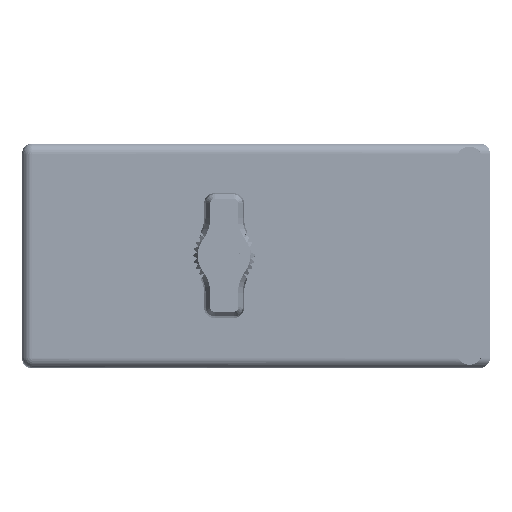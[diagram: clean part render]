
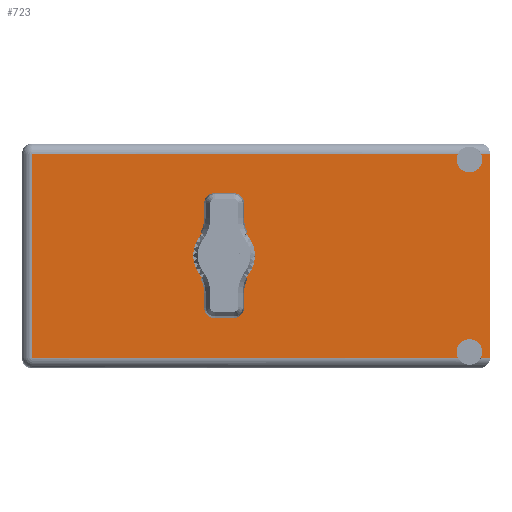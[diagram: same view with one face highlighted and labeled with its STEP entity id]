
A CAD part, top view. The second image highlights one B-rep face of the part: STEP entity #723.
In plain terms, the highlighted face is planar.
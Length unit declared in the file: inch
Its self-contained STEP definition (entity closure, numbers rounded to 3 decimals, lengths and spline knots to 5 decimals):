
#493 = LINE ( 'NONE', #103221, #78353 ) ;
#723 = ADVANCED_FACE ( 'NONE', ( #60271, #27135 ), #27679, .T. ) ;
#1004 = LINE ( 'NONE', #15747, #63517 ) ;
#2208 = EDGE_CURVE ( 'NONE', #18664, #69433, #89335, .T. ) ;
#5117 = EDGE_LOOP ( 'NONE', ( #17253, #62766 ) ) ;
#6814 = CARTESIAN_POINT ( 'NONE',  ( 1.75083, 1.93, -0.695 ) ) ;
#7413 = EDGE_CURVE ( 'NONE', #67430, #36402, #26645, .T. ) ;
#8121 = AXIS2_PLACEMENT_3D ( 'NONE', #72641, #79460, #87687 ) ;
#8572 = EDGE_CURVE ( 'NONE', #79561, #40845, #9976, .T. ) ;
#8765 = CIRCLE ( 'NONE', #11418, 0.0875 ) ;
#9651 = CARTESIAN_POINT ( 'NONE',  ( 1.75083, 1.93, 0.695 ) ) ;
#9976 = CIRCLE ( 'NONE', #65520, 0.0875 ) ;
#10219 = VECTOR ( 'NONE', #91761, 39.37008 ) ;
#11418 = AXIS2_PLACEMENT_3D ( 'NONE', #29911, #13522, #85903 ) ;
#11867 = LINE ( 'NONE', #16403, #20770 ) ;
#13522 = DIRECTION ( 'NONE',  ( 0., 1., 0. ) ) ;
#15747 = CARTESIAN_POINT ( 'NONE',  ( -1.3775, 1.93, -0.695 ) ) ;
#15960 = ORIENTED_EDGE ( 'NONE', *, *, #72037, .T. ) ;
#16130 = AXIS2_PLACEMENT_3D ( 'NONE', #52974, #28037, #84729 ) ;
#16369 = EDGE_CURVE ( 'NONE', #36402, #67430, #81219, .T. ) ;
#16403 = CARTESIAN_POINT ( 'NONE',  ( 1.8125, 1.93, 0.765 ) ) ;
#16975 = VERTEX_POINT ( 'NONE', #64319 ) ;
#17253 = ORIENTED_EDGE ( 'NONE', *, *, #7413, .F. ) ;
#18664 = VERTEX_POINT ( 'NONE', #22188 ) ;
#20640 = EDGE_CURVE ( 'NONE', #18664, #70032, #8765, .T. ) ;
#20770 = VECTOR ( 'NONE', #64906, 39.37008 ) ;
#21615 = EDGE_CURVE ( 'NONE', #89228, #28178, #76514, .T. ) ;
#21833 = CARTESIAN_POINT ( 'NONE',  ( 1.6725, 1.93, -0.656 ) ) ;
#22188 = CARTESIAN_POINT ( 'NONE',  ( 1.59417, 1.93, -0.695 ) ) ;
#23709 = DIRECTION ( 'NONE',  ( 0., 0., 1. ) ) ;
#24545 = DIRECTION ( 'NONE',  ( 0., 0., 1. ) ) ;
#26645 = CIRCLE ( 'NONE', #48939, 0.17 ) ;
#26835 = VECTOR ( 'NONE', #52426, 39.37008 ) ;
#27135 = FACE_OUTER_BOUND ( 'NONE', #100216, .T. ) ;
#27679 = PLANE ( 'NONE',  #16130 ) ;
#28037 = DIRECTION ( 'NONE',  ( 0., 1., 0. ) ) ;
#28178 = VERTEX_POINT ( 'NONE', #54635 ) ;
#28259 = CARTESIAN_POINT ( 'NONE',  ( 1.8125, 1.93, -0.695 ) ) ;
#29515 = CARTESIAN_POINT ( 'NONE',  ( -1.3075, 1.93, -0.695 ) ) ;
#29773 = AXIS2_PLACEMENT_3D ( 'NONE', #64821, #73354, #24545 ) ;
#29911 = CARTESIAN_POINT ( 'NONE',  ( 1.6725, 1.93, -0.656 ) ) ;
#31079 = DIRECTION ( 'NONE',  ( -1., 0., 0. ) ) ;
#31098 = VERTEX_POINT ( 'NONE', #6814 ) ;
#31200 = ORIENTED_EDGE ( 'NONE', *, *, #71225, .T. ) ;
#33534 = EDGE_CURVE ( 'NONE', #40845, #28178, #101100, .T. ) ;
#34710 = CARTESIAN_POINT ( 'NONE',  ( 1.8125, 1.93, 0.695 ) ) ;
#35450 = DIRECTION ( 'NONE',  ( 0., 0., 1. ) ) ;
#36167 = DIRECTION ( 'NONE',  ( 0., 1., 0. ) ) ;
#36402 = VERTEX_POINT ( 'NONE', #98772 ) ;
#37330 = EDGE_CURVE ( 'NONE', #69433, #89228, #493, .T. ) ;
#39393 = CARTESIAN_POINT ( 'NONE',  ( 1.6725, 1.93, 0.656 ) ) ;
#40845 = VERTEX_POINT ( 'NONE', #102457 ) ;
#47399 = DIRECTION ( 'NONE',  ( 0., 1., 0. ) ) ;
#47539 = DIRECTION ( 'NONE',  ( 0., 1., 0. ) ) ;
#48224 = CARTESIAN_POINT ( 'NONE',  ( 1.6725, 1.93, -0.5685 ) ) ;
#48939 = AXIS2_PLACEMENT_3D ( 'NONE', #67890, #36167, #35450 ) ;
#52426 = DIRECTION ( 'NONE',  ( -1., 0., 0. ) ) ;
#52668 = ORIENTED_EDGE ( 'NONE', *, *, #20640, .F. ) ;
#52974 = CARTESIAN_POINT ( 'NONE',  ( -1.3775, 1.93, -0.765 ) ) ;
#54635 = CARTESIAN_POINT ( 'NONE',  ( 1.59417, 1.93, 0.695 ) ) ;
#58409 = CARTESIAN_POINT ( 'NONE',  ( 1.8125, 1.93, 0.695 ) ) ;
#59192 = ORIENTED_EDGE ( 'NONE', *, *, #21615, .T. ) ;
#60271 = FACE_BOUND ( 'NONE', #5117, .T. ) ;
#62766 = ORIENTED_EDGE ( 'NONE', *, *, #16369, .F. ) ;
#62959 = DIRECTION ( 'NONE',  ( 0., 0., 1. ) ) ;
#63517 = VECTOR ( 'NONE', #31079, 39.37008 ) ;
#64319 = CARTESIAN_POINT ( 'NONE',  ( 1.8125, 1.93, 0.695 ) ) ;
#64821 = CARTESIAN_POINT ( 'NONE',  ( 0., 1.93, 0. ) ) ;
#64906 = DIRECTION ( 'NONE',  ( 0., 0., 1. ) ) ;
#65520 = AXIS2_PLACEMENT_3D ( 'NONE', #39393, #47539, #23709 ) ;
#67430 = VERTEX_POINT ( 'NONE', #70138 ) ;
#67890 = CARTESIAN_POINT ( 'NONE',  ( 0., 1.93, 0. ) ) ;
#68109 = ORIENTED_EDGE ( 'NONE', *, *, #37330, .T. ) ;
#69131 = CARTESIAN_POINT ( 'NONE',  ( -1.3775, 1.93, -0.695 ) ) ;
#69433 = VERTEX_POINT ( 'NONE', #29515 ) ;
#70032 = VERTEX_POINT ( 'NONE', #48224 ) ;
#70138 = CARTESIAN_POINT ( 'NONE',  ( 0., 1.93, 0.17 ) ) ;
#70301 = ORIENTED_EDGE ( 'NONE', *, *, #92691, .F. ) ;
#71225 = EDGE_CURVE ( 'NONE', #77256, #31098, #1004, .T. ) ;
#72037 = EDGE_CURVE ( 'NONE', #79561, #16975, #104089, .T. ) ;
#72641 = CARTESIAN_POINT ( 'NONE',  ( 1.6725, 1.93, 0.656 ) ) ;
#73354 = DIRECTION ( 'NONE',  ( 0., 1., 0. ) ) ;
#75914 = ORIENTED_EDGE ( 'NONE', *, *, #33534, .F. ) ;
#76514 = LINE ( 'NONE', #34710, #10219 ) ;
#77256 = VERTEX_POINT ( 'NONE', #28259 ) ;
#78353 = VECTOR ( 'NONE', #62959, 39.37008 ) ;
#79460 = DIRECTION ( 'NONE',  ( 0., 1., 0. ) ) ;
#79561 = VERTEX_POINT ( 'NONE', #9651 ) ;
#80917 = CARTESIAN_POINT ( 'NONE',  ( -1.3075, 1.93, 0.695 ) ) ;
#81219 = CIRCLE ( 'NONE', #29773, 0.17 ) ;
#82449 = VECTOR ( 'NONE', #99400, 39.37008 ) ;
#84069 = ORIENTED_EDGE ( 'NONE', *, *, #86771, .F. ) ;
#84729 = DIRECTION ( 'NONE',  ( -1., 0., 0. ) ) ;
#84910 = AXIS2_PLACEMENT_3D ( 'NONE', #21833, #47399, #86733 ) ;
#85684 = CIRCLE ( 'NONE', #84910, 0.0875 ) ;
#85903 = DIRECTION ( 'NONE',  ( 0., 0., 1. ) ) ;
#86733 = DIRECTION ( 'NONE',  ( 0., 0., 1. ) ) ;
#86771 = EDGE_CURVE ( 'NONE', #70032, #31098, #85684, .T. ) ;
#87687 = DIRECTION ( 'NONE',  ( 0., 0., 1. ) ) ;
#89228 = VERTEX_POINT ( 'NONE', #80917 ) ;
#89335 = LINE ( 'NONE', #69131, #26835 ) ;
#90094 = ORIENTED_EDGE ( 'NONE', *, *, #2208, .T. ) ;
#91761 = DIRECTION ( 'NONE',  ( 1., 0., 0. ) ) ;
#92691 = EDGE_CURVE ( 'NONE', #77256, #16975, #11867, .T. ) ;
#98772 = CARTESIAN_POINT ( 'NONE',  ( 0., 1.93, -0.17 ) ) ;
#98856 = ORIENTED_EDGE ( 'NONE', *, *, #8572, .F. ) ;
#99400 = DIRECTION ( 'NONE',  ( 1., 0., 0. ) ) ;
#100216 = EDGE_LOOP ( 'NONE', ( #59192, #75914, #98856, #15960, #70301, #31200, #84069, #52668, #90094, #68109 ) ) ;
#101100 = CIRCLE ( 'NONE', #8121, 0.0875 ) ;
#102457 = CARTESIAN_POINT ( 'NONE',  ( 1.6725, 1.93, 0.5685 ) ) ;
#103221 = CARTESIAN_POINT ( 'NONE',  ( -1.3075, 1.93, -0.765 ) ) ;
#104089 = LINE ( 'NONE', #58409, #82449 ) ;
